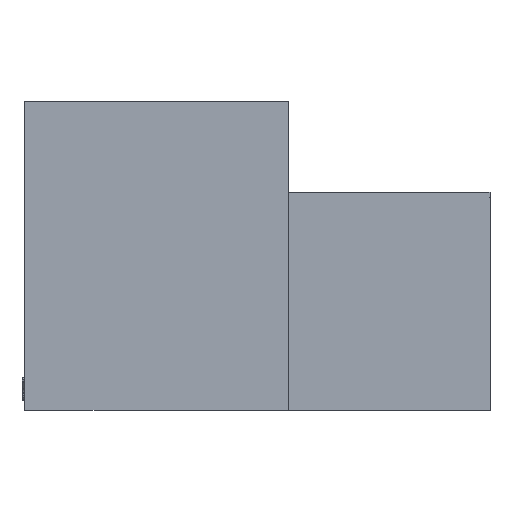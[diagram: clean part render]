
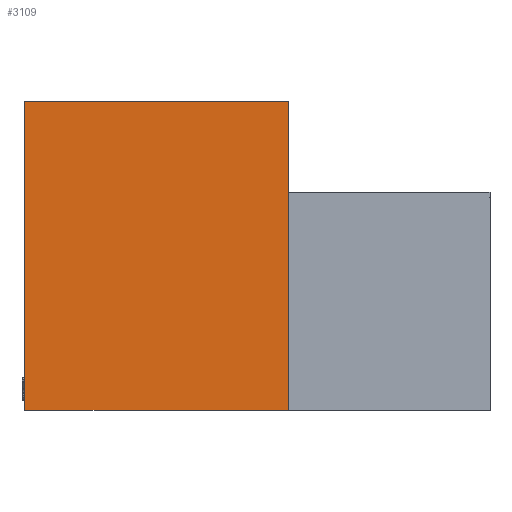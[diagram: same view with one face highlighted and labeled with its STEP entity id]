
A CAD part, left-side view. The second image highlights one B-rep face of the part: STEP entity #3109.
In plain terms, the highlighted planar face has unit normal (-1, 0, 0).
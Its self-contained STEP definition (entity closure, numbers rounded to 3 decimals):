
#1174 = DIRECTION ( 'NONE',  ( 0., 1., 0. ) ) ;
#1475 = LINE ( 'NONE', #23855, #21740 ) ;
#2651 = DIRECTION ( 'NONE',  ( 0., 0., -1. ) ) ;
#3109 = ADVANCED_FACE ( 'NONE', ( #8177 ), #3921, .F. ) ;
#3921 = PLANE ( 'NONE',  #8139 ) ;
#4046 = DIRECTION ( 'NONE',  ( 0., 0., -1. ) ) ;
#4802 = CARTESIAN_POINT ( 'NONE',  ( 0., 11.506, 0. ) ) ;
#5335 = LINE ( 'NONE', #16840, #36155 ) ;
#5417 = ORIENTED_EDGE ( 'NONE', *, *, #8711, .F. ) ;
#7107 = VERTEX_POINT ( 'NONE', #34382 ) ;
#7677 = CARTESIAN_POINT ( 'NONE',  ( 0., 0., 0. ) ) ;
#8139 = AXIS2_PLACEMENT_3D ( 'NONE', #9703, #20576, #4046 ) ;
#8177 = FACE_OUTER_BOUND ( 'NONE', #9311, .T. ) ;
#8642 = VERTEX_POINT ( 'NONE', #33819 ) ;
#8711 = EDGE_CURVE ( 'NONE', #25779, #32848, #5335, .T. ) ;
#9110 = LINE ( 'NONE', #20035, #19713 ) ;
#9156 = DIRECTION ( 'NONE',  ( 0., 0., 1. ) ) ;
#9311 = EDGE_LOOP ( 'NONE', ( #29219, #12588, #5417, #26165 ) ) ;
#9703 = CARTESIAN_POINT ( 'NONE',  ( 0., 0., 0. ) ) ;
#12588 = ORIENTED_EDGE ( 'NONE', *, *, #33076, .F. ) ;
#13144 = VECTOR ( 'NONE', #2651, 1000. ) ;
#16840 = CARTESIAN_POINT ( 'NONE',  ( 0., 11.506, 0. ) ) ;
#19713 = VECTOR ( 'NONE', #9156, 1000. ) ;
#20035 = CARTESIAN_POINT ( 'NONE',  ( 0., 11.506, -13.487 ) ) ;
#20576 = DIRECTION ( 'NONE',  ( 1., 0., 0. ) ) ;
#21740 = VECTOR ( 'NONE', #1174, 1000. ) ;
#22383 = DIRECTION ( 'NONE',  ( 0., -1., 0. ) ) ;
#23855 = CARTESIAN_POINT ( 'NONE',  ( 0., -8.814, -13.487 ) ) ;
#25440 = CARTESIAN_POINT ( 'NONE',  ( 0., 0., 0. ) ) ;
#25779 = VERTEX_POINT ( 'NONE', #4802 ) ;
#26165 = ORIENTED_EDGE ( 'NONE', *, *, #34924, .F. ) ;
#29219 = ORIENTED_EDGE ( 'NONE', *, *, #30045, .F. ) ;
#29906 = LINE ( 'NONE', #25440, #13144 ) ;
#30045 = EDGE_CURVE ( 'NONE', #8642, #7107, #1475, .T. ) ;
#32848 = VERTEX_POINT ( 'NONE', #7677 ) ;
#33076 = EDGE_CURVE ( 'NONE', #32848, #8642, #29906, .T. ) ;
#33819 = CARTESIAN_POINT ( 'NONE',  ( 0., 0., -13.487 ) ) ;
#34382 = CARTESIAN_POINT ( 'NONE',  ( 0., 11.506, -13.487 ) ) ;
#34924 = EDGE_CURVE ( 'NONE', #7107, #25779, #9110, .T. ) ;
#36155 = VECTOR ( 'NONE', #22383, 1000. ) ;
